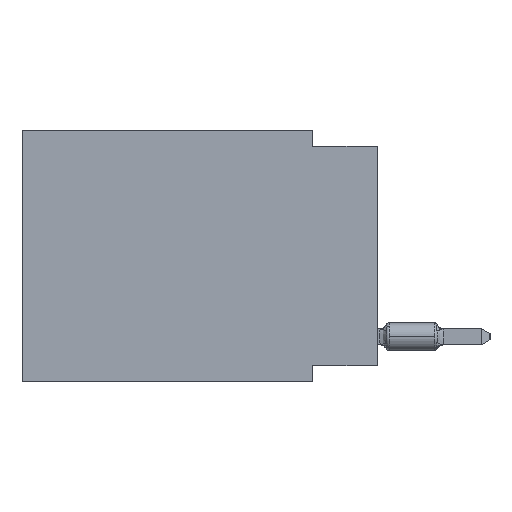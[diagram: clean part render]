
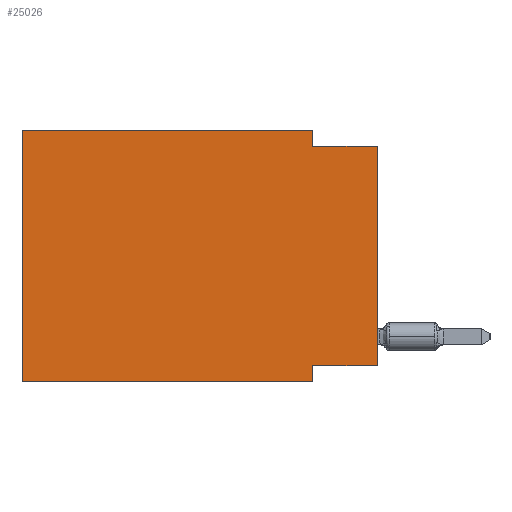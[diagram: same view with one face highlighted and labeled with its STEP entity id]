
A CAD part, left-side view. The second image highlights one B-rep face of the part: STEP entity #25026.
In plain terms, the highlighted planar face has unit normal (-1, 0, 0).
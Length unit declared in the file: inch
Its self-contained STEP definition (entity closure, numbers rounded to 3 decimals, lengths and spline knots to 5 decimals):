
#12 = EDGE_CURVE ( 'NONE', #4200, #40272, #14251, .T. ) ;
#1012 = DIRECTION ( 'NONE',  ( 0., -1., 0. ) ) ;
#1440 = AXIS2_PLACEMENT_3D ( 'NONE', #39251, #18245, #38994 ) ;
#1745 = EDGE_CURVE ( 'NONE', #35028, #40272, #40175, .T. ) ;
#3057 = EDGE_CURVE ( 'NONE', #31650, #9200, #6010, .T. ) ;
#3075 = CARTESIAN_POINT ( 'NONE',  ( 0., 0., -0.365 ) ) ;
#3359 = VERTEX_POINT ( 'NONE', #50313 ) ;
#3801 = DIRECTION ( 'NONE',  ( 0., 0., -1. ) ) ;
#3872 = ORIENTED_EDGE ( 'NONE', *, *, #36414, .F. ) ;
#4200 = VERTEX_POINT ( 'NONE', #20622 ) ;
#4320 = LINE ( 'NONE', #16510, #14134 ) ;
#4713 = CARTESIAN_POINT ( 'NONE',  ( 0., 0., -0.025 ) ) ;
#6010 = LINE ( 'NONE', #22190, #22534 ) ;
#6531 = DIRECTION ( 'NONE',  ( 0., 0., 1. ) ) ;
#7021 = VERTEX_POINT ( 'NONE', #52253 ) ;
#7913 = CARTESIAN_POINT ( 'NONE',  ( 0., 0., -0.025 ) ) ;
#8811 = VECTOR ( 'NONE', #3801, 39.37008 ) ;
#9200 = VERTEX_POINT ( 'NONE', #4713 ) ;
#9690 = VECTOR ( 'NONE', #35185, 39.37008 ) ;
#10821 = FACE_OUTER_BOUND ( 'NONE', #24124, .T. ) ;
#12793 = CARTESIAN_POINT ( 'NONE',  ( 0., 0.1, 0. ) ) ;
#14134 = VECTOR ( 'NONE', #32719, 39.37008 ) ;
#14251 = LINE ( 'NONE', #14765, #37462 ) ;
#14682 = DIRECTION ( 'NONE',  ( 0., 0., -1. ) ) ;
#14765 = CARTESIAN_POINT ( 'NONE',  ( 0., 0.55, -0.39 ) ) ;
#16510 = CARTESIAN_POINT ( 'NONE',  ( 0., 0.55, 0. ) ) ;
#17763 = EDGE_CURVE ( 'NONE', #31650, #35028, #51417, .T. ) ;
#18245 = DIRECTION ( 'NONE',  ( 1., 0., 0. ) ) ;
#18643 = CARTESIAN_POINT ( 'NONE',  ( 0., 0.1, 0. ) ) ;
#18659 = ORIENTED_EDGE ( 'NONE', *, *, #27236, .F. ) ;
#20622 = CARTESIAN_POINT ( 'NONE',  ( 0., 0.55, -0.39 ) ) ;
#21548 = DIRECTION ( 'NONE',  ( 0., 0., 1. ) ) ;
#21912 = CARTESIAN_POINT ( 'NONE',  ( 0., 0.1, -0.39 ) ) ;
#22190 = CARTESIAN_POINT ( 'NONE',  ( 0., 0., 0. ) ) ;
#22227 = DIRECTION ( 'NONE',  ( 0., -1., 0. ) ) ;
#22534 = VECTOR ( 'NONE', #6531, 39.37008 ) ;
#23290 = PLANE ( 'NONE',  #1440 ) ;
#24124 = EDGE_LOOP ( 'NONE', ( #30865, #3872, #43626, #18659, #25838, #35534, #32074, #38673 ) ) ;
#25006 = CARTESIAN_POINT ( 'NONE',  ( 0., 0.55, 0. ) ) ;
#25026 = ADVANCED_FACE ( 'NONE', ( #10821 ), #23290, .F. ) ;
#25838 = ORIENTED_EDGE ( 'NONE', *, *, #27267, .F. ) ;
#27236 = EDGE_CURVE ( 'NONE', #3359, #34180, #4320, .T. ) ;
#27267 = EDGE_CURVE ( 'NONE', #4200, #3359, #41476, .T. ) ;
#28472 = CARTESIAN_POINT ( 'NONE',  ( 0., 0.1, -0.39 ) ) ;
#30865 = ORIENTED_EDGE ( 'NONE', *, *, #3057, .T. ) ;
#31650 = VERTEX_POINT ( 'NONE', #36685 ) ;
#32074 = ORIENTED_EDGE ( 'NONE', *, *, #1745, .F. ) ;
#32719 = DIRECTION ( 'NONE',  ( 0., -1., 0. ) ) ;
#34180 = VERTEX_POINT ( 'NONE', #12793 ) ;
#35028 = VERTEX_POINT ( 'NONE', #45559 ) ;
#35185 = DIRECTION ( 'NONE',  ( 0., 1., 0. ) ) ;
#35534 = ORIENTED_EDGE ( 'NONE', *, *, #12, .T. ) ;
#36414 = EDGE_CURVE ( 'NONE', #7021, #9200, #41103, .T. ) ;
#36685 = CARTESIAN_POINT ( 'NONE',  ( 0., 0., -0.365 ) ) ;
#37462 = VECTOR ( 'NONE', #22227, 39.37008 ) ;
#38673 = ORIENTED_EDGE ( 'NONE', *, *, #17763, .F. ) ;
#38881 = LINE ( 'NONE', #18643, #46431 ) ;
#38994 = DIRECTION ( 'NONE',  ( 0., 0., -1. ) ) ;
#39251 = CARTESIAN_POINT ( 'NONE',  ( 0., 0.55, 0. ) ) ;
#40175 = LINE ( 'NONE', #28472, #8811 ) ;
#40272 = VERTEX_POINT ( 'NONE', #21912 ) ;
#41103 = LINE ( 'NONE', #7913, #45244 ) ;
#41476 = LINE ( 'NONE', #25006, #49811 ) ;
#43626 = ORIENTED_EDGE ( 'NONE', *, *, #49997, .F. ) ;
#45244 = VECTOR ( 'NONE', #1012, 39.37008 ) ;
#45559 = CARTESIAN_POINT ( 'NONE',  ( 0., 0.1, -0.365 ) ) ;
#46431 = VECTOR ( 'NONE', #14682, 39.37008 ) ;
#49811 = VECTOR ( 'NONE', #21548, 39.37008 ) ;
#49997 = EDGE_CURVE ( 'NONE', #34180, #7021, #38881, .T. ) ;
#50313 = CARTESIAN_POINT ( 'NONE',  ( 0., 0.55, 0. ) ) ;
#51417 = LINE ( 'NONE', #3075, #9690 ) ;
#52253 = CARTESIAN_POINT ( 'NONE',  ( 0., 0.1, -0.025 ) ) ;
